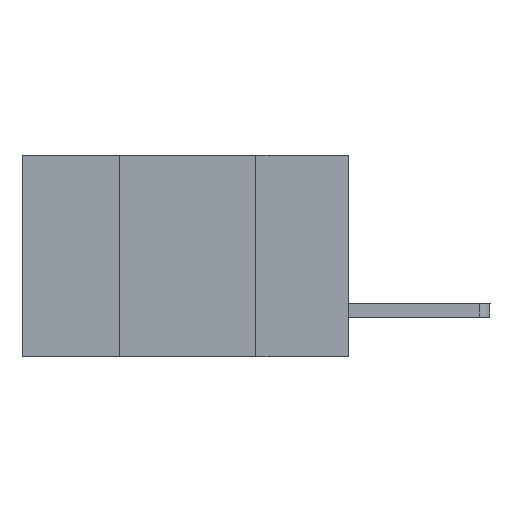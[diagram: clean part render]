
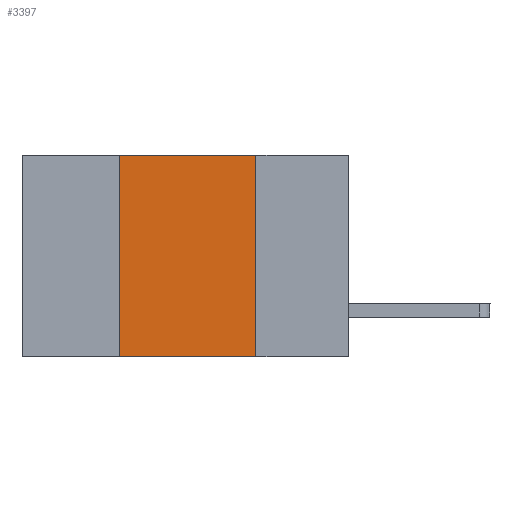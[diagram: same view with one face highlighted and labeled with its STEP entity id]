
A CAD part, left-side view. The second image highlights one B-rep face of the part: STEP entity #3397.
In plain terms, the highlighted planar face has unit normal (-1, 0, 0).
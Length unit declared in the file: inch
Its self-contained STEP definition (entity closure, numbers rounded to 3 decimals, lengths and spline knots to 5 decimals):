
#68 = EDGE_CURVE ( 'NONE', #3947, #6572, #2370, .T. ) ;
#591 = ORIENTED_EDGE ( 'NONE', *, *, #6079, .T. ) ;
#745 = DIRECTION ( 'NONE',  ( 1., 0., 0. ) ) ;
#903 = CARTESIAN_POINT ( 'NONE',  ( 0., 0.17, -0.37 ) ) ;
#2370 = LINE ( 'NONE', #4826, #8645 ) ;
#2554 = EDGE_CURVE ( 'NONE', #4806, #3405, #4056, .T. ) ;
#3023 = VECTOR ( 'NONE', #10555, 39.37008 ) ;
#3056 = VECTOR ( 'NONE', #8237, 39.37008 ) ;
#3156 = CARTESIAN_POINT ( 'NONE',  ( 0., 0.6, 0. ) ) ;
#3232 = VECTOR ( 'NONE', #3440, 39.37008 ) ;
#3397 = ADVANCED_FACE ( 'NONE', ( #10511 ), #10463, .F. ) ;
#3405 = VERTEX_POINT ( 'NONE', #5668 ) ;
#3440 = DIRECTION ( 'NONE',  ( 0., -1., 0. ) ) ;
#3947 = VERTEX_POINT ( 'NONE', #5283 ) ;
#4056 = LINE ( 'NONE', #903, #3023 ) ;
#4232 = CARTESIAN_POINT ( 'NONE',  ( 0., 0.17, 0. ) ) ;
#4688 = ORIENTED_EDGE ( 'NONE', *, *, #2554, .F. ) ;
#4806 = VERTEX_POINT ( 'NONE', #4232 ) ;
#4826 = CARTESIAN_POINT ( 'NONE',  ( 0., 0.42, -0.37 ) ) ;
#4930 = CARTESIAN_POINT ( 'NONE',  ( 0., 0.6, 0. ) ) ;
#5283 = CARTESIAN_POINT ( 'NONE',  ( 0., 0.42, -0.37 ) ) ;
#5668 = CARTESIAN_POINT ( 'NONE',  ( 0., 0.17, -0.37 ) ) ;
#5682 = CARTESIAN_POINT ( 'NONE',  ( 0., 0.6, -0.37 ) ) ;
#5782 = EDGE_LOOP ( 'NONE', ( #4688, #10329, #9488, #591 ) ) ;
#6079 = EDGE_CURVE ( 'NONE', #3947, #3405, #7377, .T. ) ;
#6144 = EDGE_CURVE ( 'NONE', #6572, #4806, #9103, .T. ) ;
#6572 = VERTEX_POINT ( 'NONE', #10240 ) ;
#7250 = DIRECTION ( 'NONE',  ( 0., 0., -1. ) ) ;
#7377 = LINE ( 'NONE', #5682, #3056 ) ;
#8237 = DIRECTION ( 'NONE',  ( 0., -1., 0. ) ) ;
#8645 = VECTOR ( 'NONE', #10321, 39.37008 ) ;
#8837 = AXIS2_PLACEMENT_3D ( 'NONE', #3156, #745, #7250 ) ;
#9103 = LINE ( 'NONE', #4930, #3232 ) ;
#9488 = ORIENTED_EDGE ( 'NONE', *, *, #68, .F. ) ;
#10240 = CARTESIAN_POINT ( 'NONE',  ( 0., 0.42, 0. ) ) ;
#10321 = DIRECTION ( 'NONE',  ( 0., 0., 1. ) ) ;
#10329 = ORIENTED_EDGE ( 'NONE', *, *, #6144, .F. ) ;
#10463 = PLANE ( 'NONE',  #8837 ) ;
#10511 = FACE_OUTER_BOUND ( 'NONE', #5782, .T. ) ;
#10555 = DIRECTION ( 'NONE',  ( 0., 0., -1. ) ) ;
